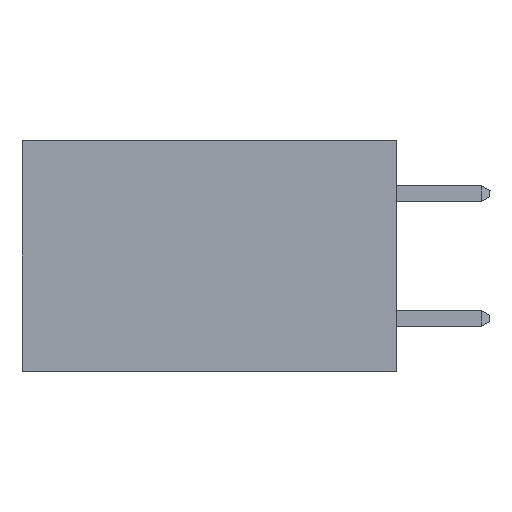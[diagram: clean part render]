
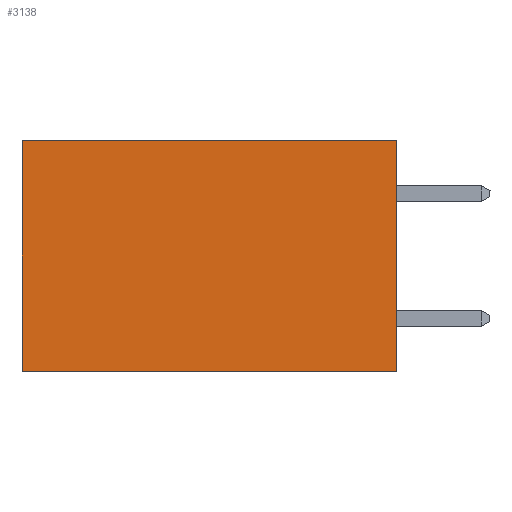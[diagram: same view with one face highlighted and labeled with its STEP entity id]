
A CAD part, left-side view. The second image highlights one B-rep face of the part: STEP entity #3138.
In plain terms, the highlighted planar face has unit normal (-1, 0, 0).
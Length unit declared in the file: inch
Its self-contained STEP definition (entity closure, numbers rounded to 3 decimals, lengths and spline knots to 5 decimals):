
#150 = EDGE_LOOP ( 'NONE', ( #8652, #6201, #8958, #853 ) ) ;
#160 = CARTESIAN_POINT ( 'NONE',  ( 0.298, 0., 0. ) ) ;
#853 = ORIENTED_EDGE ( 'NONE', *, *, #6636, .T. ) ;
#874 = FACE_OUTER_BOUND ( 'NONE', #150, .T. ) ;
#3138 = ADVANCED_FACE ( 'NONE', ( #874 ), #4685, .F. ) ;
#3254 = CARTESIAN_POINT ( 'NONE',  ( 0.298, 0., -0.37 ) ) ;
#4179 = EDGE_CURVE ( 'NONE', #10506, #7846, #9101, .T. ) ;
#4685 = PLANE ( 'NONE',  #8267 ) ;
#4799 = LINE ( 'NONE', #4858, #12745 ) ;
#4858 = CARTESIAN_POINT ( 'NONE',  ( 0.298, 0., 0. ) ) ;
#4953 = DIRECTION ( 'NONE',  ( 0., 1., 0. ) ) ;
#6152 = DIRECTION ( 'NONE',  ( 1., 0., 0. ) ) ;
#6172 = LINE ( 'NONE', #10643, #11608 ) ;
#6201 = ORIENTED_EDGE ( 'NONE', *, *, #10849, .F. ) ;
#6636 = EDGE_CURVE ( 'NONE', #10506, #8858, #4799, .T. ) ;
#7846 = VERTEX_POINT ( 'NONE', #10928 ) ;
#8267 = AXIS2_PLACEMENT_3D ( 'NONE', #160, #6152, #13239 ) ;
#8652 = ORIENTED_EDGE ( 'NONE', *, *, #8659, .T. ) ;
#8659 = EDGE_CURVE ( 'NONE', #8858, #13191, #6172, .T. ) ;
#8798 = VECTOR ( 'NONE', #12637, 39.37008 ) ;
#8858 = VERTEX_POINT ( 'NONE', #8979 ) ;
#8958 = ORIENTED_EDGE ( 'NONE', *, *, #4179, .F. ) ;
#8979 = CARTESIAN_POINT ( 'NONE',  ( 0.298, 0.6, 0. ) ) ;
#9101 = LINE ( 'NONE', #10147, #8798 ) ;
#10090 = LINE ( 'NONE', #3254, #10392 ) ;
#10147 = CARTESIAN_POINT ( 'NONE',  ( 0.298, 0., 0. ) ) ;
#10392 = VECTOR ( 'NONE', #10469, 39.37008 ) ;
#10469 = DIRECTION ( 'NONE',  ( 0., 1., 0. ) ) ;
#10506 = VERTEX_POINT ( 'NONE', #13125 ) ;
#10643 = CARTESIAN_POINT ( 'NONE',  ( 0.298, 0.6, 0. ) ) ;
#10661 = DIRECTION ( 'NONE',  ( 0., 0., -1. ) ) ;
#10849 = EDGE_CURVE ( 'NONE', #7846, #13191, #10090, .T. ) ;
#10907 = CARTESIAN_POINT ( 'NONE',  ( 0.298, 0.6, -0.37 ) ) ;
#10928 = CARTESIAN_POINT ( 'NONE',  ( 0.298, 0., -0.37 ) ) ;
#11608 = VECTOR ( 'NONE', #10661, 39.37008 ) ;
#12637 = DIRECTION ( 'NONE',  ( 0., 0., -1. ) ) ;
#12745 = VECTOR ( 'NONE', #4953, 39.37008 ) ;
#13125 = CARTESIAN_POINT ( 'NONE',  ( 0.298, 0., 0. ) ) ;
#13191 = VERTEX_POINT ( 'NONE', #10907 ) ;
#13239 = DIRECTION ( 'NONE',  ( 0., 0., -1. ) ) ;
